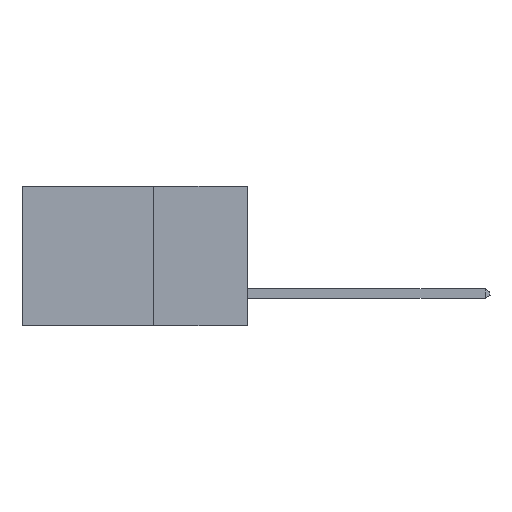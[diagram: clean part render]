
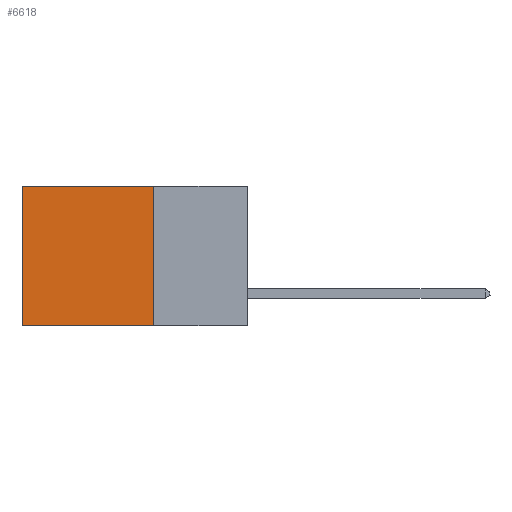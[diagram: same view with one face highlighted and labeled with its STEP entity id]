
A CAD part, left-side view. The second image highlights one B-rep face of the part: STEP entity #6618.
In plain terms, the highlighted planar face has unit normal (-1, 0, 0).
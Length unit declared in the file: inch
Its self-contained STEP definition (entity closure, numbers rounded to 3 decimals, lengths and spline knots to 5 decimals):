
#315 = DIRECTION ( 'NONE',  ( 0., 0., -1. ) ) ;
#774 = AXIS2_PLACEMENT_3D ( 'NONE', #1934, #5073, #19150 ) ;
#1018 = EDGE_CURVE ( 'NONE', #6466, #3558, #15946, .T. ) ;
#1934 = CARTESIAN_POINT ( 'NONE',  ( 0.298, 0.25, 0. ) ) ;
#2343 = EDGE_CURVE ( 'NONE', #18310, #6466, #11338, .T. ) ;
#2635 = EDGE_LOOP ( 'NONE', ( #7388, #5691, #18969, #12712 ) ) ;
#3558 = VERTEX_POINT ( 'NONE', #11555 ) ;
#4256 = VECTOR ( 'NONE', #5936, 39.37008 ) ;
#5073 = DIRECTION ( 'NONE',  ( 1., 0., 0. ) ) ;
#5691 = ORIENTED_EDGE ( 'NONE', *, *, #1018, .F. ) ;
#5936 = DIRECTION ( 'NONE',  ( 0., 1., 0. ) ) ;
#6466 = VERTEX_POINT ( 'NONE', #15538 ) ;
#6618 = ADVANCED_FACE ( 'NONE', ( #7692 ), #12762, .F. ) ;
#7388 = ORIENTED_EDGE ( 'NONE', *, *, #15745, .T. ) ;
#7692 = FACE_OUTER_BOUND ( 'NONE', #2635, .T. ) ;
#8043 = DIRECTION ( 'NONE',  ( 0., 0., -1. ) ) ;
#9474 = LINE ( 'NONE', #18836, #11437 ) ;
#10833 = VERTEX_POINT ( 'NONE', #14228 ) ;
#11338 = LINE ( 'NONE', #11444, #12073 ) ;
#11437 = VECTOR ( 'NONE', #8043, 39.37008 ) ;
#11444 = CARTESIAN_POINT ( 'NONE',  ( 0.298, 0.25, 0. ) ) ;
#11471 = CARTESIAN_POINT ( 'NONE',  ( 0.298, 0.25, 0. ) ) ;
#11555 = CARTESIAN_POINT ( 'NONE',  ( 0.298, 0.6, -0.37 ) ) ;
#11812 = VECTOR ( 'NONE', #17062, 39.37008 ) ;
#12073 = VECTOR ( 'NONE', #315, 39.37008 ) ;
#12712 = ORIENTED_EDGE ( 'NONE', *, *, #12799, .T. ) ;
#12762 = PLANE ( 'NONE',  #774 ) ;
#12799 = EDGE_CURVE ( 'NONE', #18310, #10833, #14243, .T. ) ;
#14228 = CARTESIAN_POINT ( 'NONE',  ( 0.298, 0.6, 0. ) ) ;
#14243 = LINE ( 'NONE', #16953, #4256 ) ;
#15476 = CARTESIAN_POINT ( 'NONE',  ( 0.298, 0.25, -0.37 ) ) ;
#15538 = CARTESIAN_POINT ( 'NONE',  ( 0.298, 0.25, -0.37 ) ) ;
#15745 = EDGE_CURVE ( 'NONE', #10833, #3558, #9474, .T. ) ;
#15946 = LINE ( 'NONE', #15476, #11812 ) ;
#16953 = CARTESIAN_POINT ( 'NONE',  ( 0.298, 0.25, 0. ) ) ;
#17062 = DIRECTION ( 'NONE',  ( 0., 1., 0. ) ) ;
#18310 = VERTEX_POINT ( 'NONE', #11471 ) ;
#18836 = CARTESIAN_POINT ( 'NONE',  ( 0.298, 0.6, 0. ) ) ;
#18969 = ORIENTED_EDGE ( 'NONE', *, *, #2343, .F. ) ;
#19150 = DIRECTION ( 'NONE',  ( 0., 0., -1. ) ) ;
